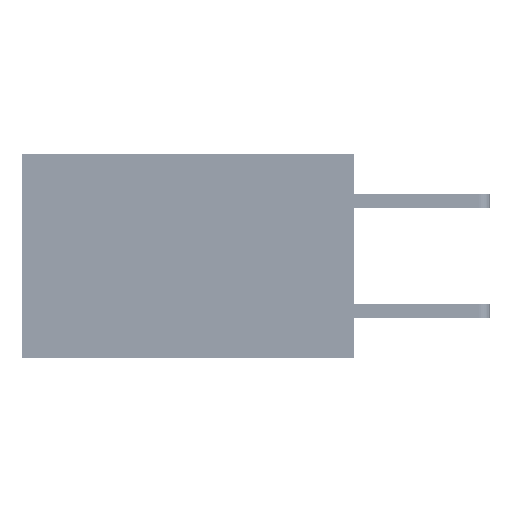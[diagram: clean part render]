
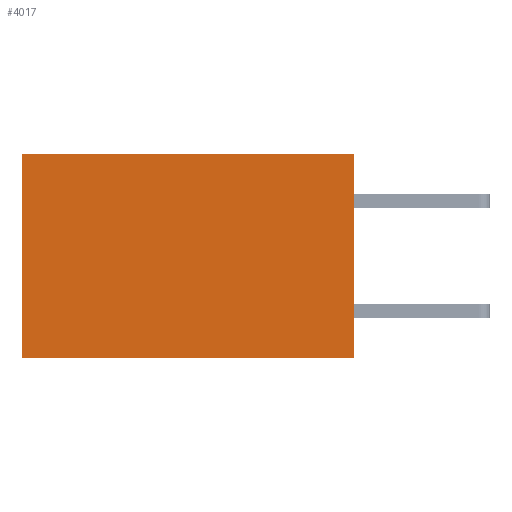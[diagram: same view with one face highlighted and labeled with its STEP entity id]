
A CAD part, left-side view. The second image highlights one B-rep face of the part: STEP entity #4017.
In plain terms, the highlighted planar face has unit normal (-1, 0, 0).
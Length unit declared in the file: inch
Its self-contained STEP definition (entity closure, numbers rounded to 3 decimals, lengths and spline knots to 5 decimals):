
#274 = VECTOR ( 'NONE', #39780, 39.37008 ) ;
#1963 = CARTESIAN_POINT ( 'NONE',  ( 0.2875, 0., -0.37 ) ) ;
#3104 = DIRECTION ( 'NONE',  ( 1., 0., 0. ) ) ;
#3655 = CARTESIAN_POINT ( 'NONE',  ( 0.2875, 0., -0.37 ) ) ;
#3662 = EDGE_CURVE ( 'NONE', #47343, #44232, #7522, .T. ) ;
#4017 = ADVANCED_FACE ( 'NONE', ( #7725 ), #38373, .F. ) ;
#5028 = EDGE_LOOP ( 'NONE', ( #26779, #26815, #17204, #12021 ) ) ;
#5524 = LINE ( 'NONE', #17380, #8770 ) ;
#6550 = AXIS2_PLACEMENT_3D ( 'NONE', #19057, #3104, #30887 ) ;
#7123 = CARTESIAN_POINT ( 'NONE',  ( 0.2875, 0.6, -0.37 ) ) ;
#7522 = LINE ( 'NONE', #3655, #39797 ) ;
#7725 = FACE_OUTER_BOUND ( 'NONE', #5028, .T. ) ;
#8111 = CARTESIAN_POINT ( 'NONE',  ( 0.2875, 0.6, 0. ) ) ;
#8770 = VECTOR ( 'NONE', #33079, 39.37008 ) ;
#10488 = EDGE_CURVE ( 'NONE', #45189, #44232, #31537, .T. ) ;
#10886 = DIRECTION ( 'NONE',  ( 0., 1., 0. ) ) ;
#12021 = ORIENTED_EDGE ( 'NONE', *, *, #29308, .T. ) ;
#17204 = ORIENTED_EDGE ( 'NONE', *, *, #27371, .F. ) ;
#17380 = CARTESIAN_POINT ( 'NONE',  ( 0.2875, 0., 0. ) ) ;
#19057 = CARTESIAN_POINT ( 'NONE',  ( 0.2875, 0., 0. ) ) ;
#19145 = VERTEX_POINT ( 'NONE', #30315 ) ;
#26779 = ORIENTED_EDGE ( 'NONE', *, *, #10488, .T. ) ;
#26815 = ORIENTED_EDGE ( 'NONE', *, *, #3662, .F. ) ;
#27371 = EDGE_CURVE ( 'NONE', #19145, #47343, #5524, .T. ) ;
#29308 = EDGE_CURVE ( 'NONE', #19145, #45189, #32265, .T. ) ;
#30315 = CARTESIAN_POINT ( 'NONE',  ( 0.2875, 0., 0. ) ) ;
#30887 = DIRECTION ( 'NONE',  ( 0., 0., -1. ) ) ;
#31537 = LINE ( 'NONE', #8111, #274 ) ;
#32265 = LINE ( 'NONE', #43859, #35872 ) ;
#33079 = DIRECTION ( 'NONE',  ( 0., 0., -1. ) ) ;
#34297 = CARTESIAN_POINT ( 'NONE',  ( 0.2875, 0.6, 0. ) ) ;
#35872 = VECTOR ( 'NONE', #40514, 39.37008 ) ;
#38373 = PLANE ( 'NONE',  #6550 ) ;
#39780 = DIRECTION ( 'NONE',  ( 0., 0., -1. ) ) ;
#39797 = VECTOR ( 'NONE', #10886, 39.37008 ) ;
#40514 = DIRECTION ( 'NONE',  ( 0., 1., 0. ) ) ;
#43859 = CARTESIAN_POINT ( 'NONE',  ( 0.2875, 0., 0. ) ) ;
#44232 = VERTEX_POINT ( 'NONE', #7123 ) ;
#45189 = VERTEX_POINT ( 'NONE', #34297 ) ;
#47343 = VERTEX_POINT ( 'NONE', #1963 ) ;
